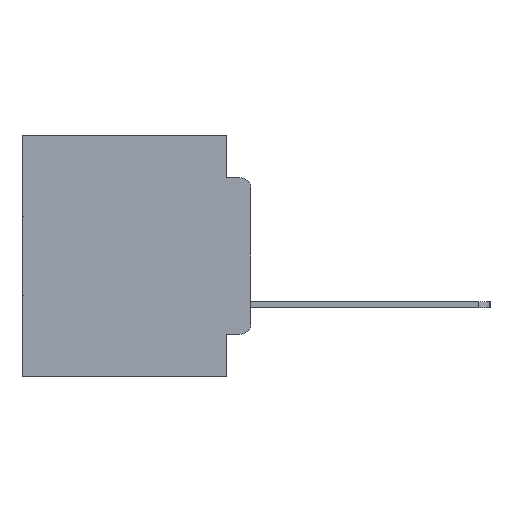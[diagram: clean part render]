
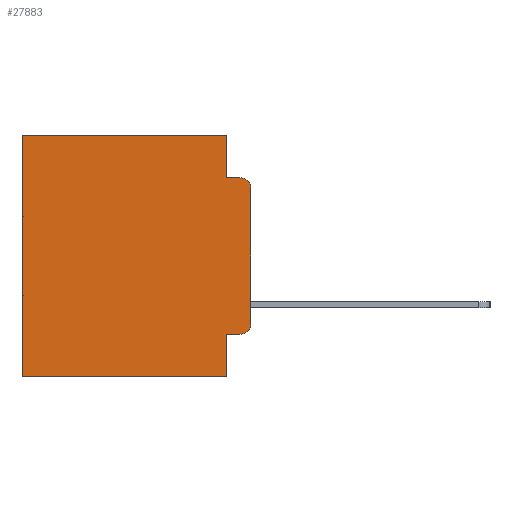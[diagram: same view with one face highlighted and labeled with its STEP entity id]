
A CAD part, left-side view. The second image highlights one B-rep face of the part: STEP entity #27883.
In plain terms, the highlighted planar face has unit normal (-1, 0, 0).
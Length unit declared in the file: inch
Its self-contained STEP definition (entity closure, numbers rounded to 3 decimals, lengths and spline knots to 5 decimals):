
#817 = EDGE_CURVE ( 'NONE', #18183, #23287, #23895, .T. ) ;
#1360 = ORIENTED_EDGE ( 'NONE', *, *, #23015, .T. ) ;
#1374 = DIRECTION ( 'NONE',  ( -1., 0., 0. ) ) ;
#1828 = VERTEX_POINT ( 'NONE', #21081 ) ;
#2127 = CARTESIAN_POINT ( 'NONE',  ( 0.298, 0.02, -0.0885 ) ) ;
#2523 = EDGE_CURVE ( 'NONE', #17553, #21624, #22682, .T. ) ;
#2536 = ORIENTED_EDGE ( 'NONE', *, *, #2523, .F. ) ;
#2729 = CARTESIAN_POINT ( 'NONE',  ( 0.298, 0.473, 0. ) ) ;
#2897 = ORIENTED_EDGE ( 'NONE', *, *, #22168, .T. ) ;
#2986 = ORIENTED_EDGE ( 'NONE', *, *, #817, .T. ) ;
#3152 = FACE_OUTER_BOUND ( 'NONE', #16564, .T. ) ;
#3359 = VECTOR ( 'NONE', #3758, 39.37008 ) ;
#3368 = CARTESIAN_POINT ( 'NONE',  ( 0.298, 0., -0.3915 ) ) ;
#3468 = CARTESIAN_POINT ( 'NONE',  ( 0.298, 0., 0. ) ) ;
#3758 = DIRECTION ( 'NONE',  ( 0., -1., 0. ) ) ;
#3909 = CARTESIAN_POINT ( 'NONE',  ( 0.298, 0., 0. ) ) ;
#5472 = VECTOR ( 'NONE', #26933, 39.37008 ) ;
#5506 = AXIS2_PLACEMENT_3D ( 'NONE', #15787, #1374, #18097 ) ;
#5621 = VECTOR ( 'NONE', #21992, 39.37008 ) ;
#5958 = LINE ( 'NONE', #18811, #23905 ) ;
#6022 = VERTEX_POINT ( 'NONE', #20878 ) ;
#6190 = CARTESIAN_POINT ( 'NONE',  ( 0.298, 0.473, 0. ) ) ;
#6194 = VERTEX_POINT ( 'NONE', #19440 ) ;
#7515 = AXIS2_PLACEMENT_3D ( 'NONE', #11066, #27176, #13429 ) ;
#7624 = ORIENTED_EDGE ( 'NONE', *, *, #18475, .T. ) ;
#8832 = PLANE ( 'NONE',  #22968 ) ;
#9148 = CARTESIAN_POINT ( 'NONE',  ( 0.298, 0.473, -0.5 ) ) ;
#9162 = DIRECTION ( 'NONE',  ( 0., 0., -1. ) ) ;
#10642 = CIRCLE ( 'NONE', #5506, 0.02 ) ;
#10711 = EDGE_CURVE ( 'NONE', #21624, #15952, #17777, .T. ) ;
#10970 = CARTESIAN_POINT ( 'NONE',  ( 0.298, 0.051, -0.4115 ) ) ;
#11066 = CARTESIAN_POINT ( 'NONE',  ( 0.298, 0.02, -0.3915 ) ) ;
#11107 = CIRCLE ( 'NONE', #7515, 0.02 ) ;
#11218 = DIRECTION ( 'NONE',  ( 0., 0., -1. ) ) ;
#11996 = LINE ( 'NONE', #26458, #5621 ) ;
#12422 = ORIENTED_EDGE ( 'NONE', *, *, #27703, .F. ) ;
#12607 = LINE ( 'NONE', #3468, #5472 ) ;
#12917 = VERTEX_POINT ( 'NONE', #27918 ) ;
#13429 = DIRECTION ( 'NONE',  ( 0., 0., -1. ) ) ;
#13800 = CARTESIAN_POINT ( 'NONE',  ( 0.298, 0.051, 0. ) ) ;
#14160 = DIRECTION ( 'NONE',  ( 0., 1., 0. ) ) ;
#14400 = EDGE_CURVE ( 'NONE', #12917, #15672, #11107, .T. ) ;
#14512 = CARTESIAN_POINT ( 'NONE',  ( 0.298, 0.051, 0. ) ) ;
#15672 = VERTEX_POINT ( 'NONE', #3368 ) ;
#15787 = CARTESIAN_POINT ( 'NONE',  ( 0.298, 0.02, -0.1085 ) ) ;
#15952 = VERTEX_POINT ( 'NONE', #2127 ) ;
#16433 = ORIENTED_EDGE ( 'NONE', *, *, #23395, .F. ) ;
#16522 = VECTOR ( 'NONE', #9162, 39.37008 ) ;
#16564 = EDGE_LOOP ( 'NONE', ( #12422, #7624, #24376, #2536, #1360, #2986, #16433, #27582, #2897, #29885 ) ) ;
#17553 = VERTEX_POINT ( 'NONE', #14512 ) ;
#17777 = LINE ( 'NONE', #20134, #29178 ) ;
#18075 = LINE ( 'NONE', #19793, #29461 ) ;
#18097 = DIRECTION ( 'NONE',  ( 0., 0., -1. ) ) ;
#18183 = VERTEX_POINT ( 'NONE', #2729 ) ;
#18475 = EDGE_CURVE ( 'NONE', #1828, #15952, #10642, .T. ) ;
#18811 = CARTESIAN_POINT ( 'NONE',  ( 0.298, 0., -0.5 ) ) ;
#19440 = CARTESIAN_POINT ( 'NONE',  ( 0.298, 0.051, -0.5 ) ) ;
#19793 = CARTESIAN_POINT ( 'NONE',  ( 0.298, 0.051, 0. ) ) ;
#20134 = CARTESIAN_POINT ( 'NONE',  ( 0.298, 0.051, -0.0885 ) ) ;
#20217 = DIRECTION ( 'NONE',  ( 0., 0., -1. ) ) ;
#20248 = DIRECTION ( 'NONE',  ( 0., -1., 0. ) ) ;
#20878 = CARTESIAN_POINT ( 'NONE',  ( 0.298, 0.051, -0.4115 ) ) ;
#21081 = CARTESIAN_POINT ( 'NONE',  ( 0.298, 0., -0.1085 ) ) ;
#21624 = VERTEX_POINT ( 'NONE', #25252 ) ;
#21992 = DIRECTION ( 'NONE',  ( 0., 1., 0. ) ) ;
#22168 = EDGE_CURVE ( 'NONE', #6022, #12917, #22939, .T. ) ;
#22682 = LINE ( 'NONE', #13800, #16522 ) ;
#22939 = LINE ( 'NONE', #10970, #3359 ) ;
#22968 = AXIS2_PLACEMENT_3D ( 'NONE', #3909, #25052, #11218 ) ;
#23015 = EDGE_CURVE ( 'NONE', #17553, #18183, #11996, .T. ) ;
#23287 = VERTEX_POINT ( 'NONE', #9148 ) ;
#23395 = EDGE_CURVE ( 'NONE', #6194, #23287, #5958, .T. ) ;
#23721 = EDGE_CURVE ( 'NONE', #6022, #6194, #18075, .T. ) ;
#23895 = LINE ( 'NONE', #6190, #29117 ) ;
#23905 = VECTOR ( 'NONE', #14160, 39.37008 ) ;
#24376 = ORIENTED_EDGE ( 'NONE', *, *, #10711, .F. ) ;
#25052 = DIRECTION ( 'NONE',  ( 1., 0., 0. ) ) ;
#25252 = CARTESIAN_POINT ( 'NONE',  ( 0.298, 0.051, -0.0885 ) ) ;
#26458 = CARTESIAN_POINT ( 'NONE',  ( 0.298, 0., 0. ) ) ;
#26933 = DIRECTION ( 'NONE',  ( 0., 0., -1. ) ) ;
#27176 = DIRECTION ( 'NONE',  ( -1., 0., 0. ) ) ;
#27582 = ORIENTED_EDGE ( 'NONE', *, *, #23721, .F. ) ;
#27703 = EDGE_CURVE ( 'NONE', #1828, #15672, #12607, .T. ) ;
#27883 = ADVANCED_FACE ( 'NONE', ( #3152 ), #8832, .F. ) ;
#27918 = CARTESIAN_POINT ( 'NONE',  ( 0.298, 0.02, -0.4115 ) ) ;
#28824 = DIRECTION ( 'NONE',  ( 0., 0., -1. ) ) ;
#29117 = VECTOR ( 'NONE', #20217, 39.37008 ) ;
#29178 = VECTOR ( 'NONE', #20248, 39.37008 ) ;
#29461 = VECTOR ( 'NONE', #28824, 39.37008 ) ;
#29885 = ORIENTED_EDGE ( 'NONE', *, *, #14400, .T. ) ;
